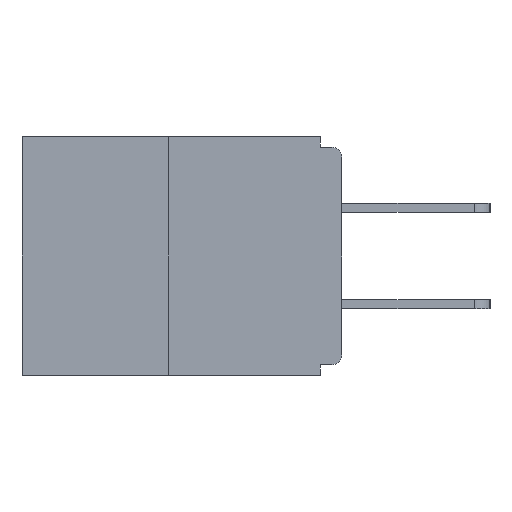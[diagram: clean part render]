
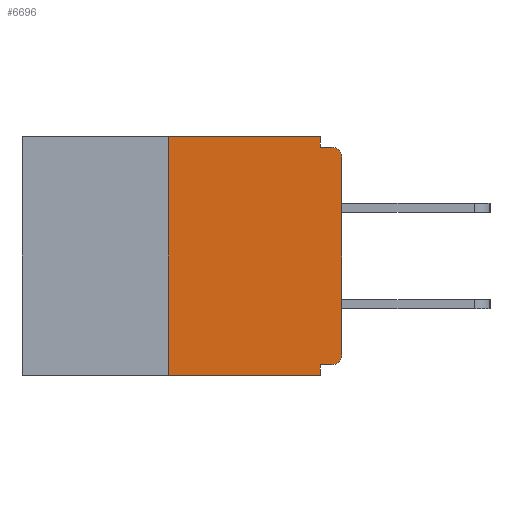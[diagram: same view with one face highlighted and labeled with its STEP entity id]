
A CAD part, left-side view. The second image highlights one B-rep face of the part: STEP entity #6696.
In plain terms, the highlighted planar face has unit normal (-1, 0, 0).
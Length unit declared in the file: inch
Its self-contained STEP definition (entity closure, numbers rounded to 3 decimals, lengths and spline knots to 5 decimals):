
#80 = FACE_OUTER_BOUND ( 'NONE', #8025, .T. ) ;
#126 = AXIS2_PLACEMENT_3D ( 'NONE', #13518, #20785, #20862 ) ;
#1583 = VECTOR ( 'NONE', #13262, 39.37008 ) ;
#1648 = EDGE_CURVE ( 'NONE', #8366, #12127, #14051, .T. ) ;
#1692 = CARTESIAN_POINT ( 'NONE',  ( 0., 0.031, -0.343 ) ) ;
#2750 = CIRCLE ( 'NONE', #5619, 0.015 ) ;
#3290 = LINE ( 'NONE', #3597, #17749 ) ;
#3597 = CARTESIAN_POINT ( 'NONE',  ( 0., 0.46, 0. ) ) ;
#3737 = CARTESIAN_POINT ( 'NONE',  ( 0., 0.25, 0. ) ) ;
#4111 = DIRECTION ( 'NONE',  ( 0., 0., 1. ) ) ;
#4221 = ORIENTED_EDGE ( 'NONE', *, *, #6422, .T. ) ;
#4353 = VECTOR ( 'NONE', #4111, 39.37008 ) ;
#4705 = VECTOR ( 'NONE', #17121, 39.37008 ) ;
#5236 = DIRECTION ( 'NONE',  ( 0., 1., 0. ) ) ;
#5619 = AXIS2_PLACEMENT_3D ( 'NONE', #15992, #16230, #19916 ) ;
#6003 = CARTESIAN_POINT ( 'NONE',  ( 0., 0., -0.03 ) ) ;
#6129 = CARTESIAN_POINT ( 'NONE',  ( 0., 0.031, 0. ) ) ;
#6188 = DIRECTION ( 'NONE',  ( 1., 0., 0. ) ) ;
#6380 = ORIENTED_EDGE ( 'NONE', *, *, #18710, .T. ) ;
#6422 = EDGE_CURVE ( 'NONE', #10304, #13069, #2750, .T. ) ;
#6431 = LINE ( 'NONE', #13459, #4353 ) ;
#6696 = ADVANCED_FACE ( 'NONE', ( #80 ), #14452, .F. ) ;
#7103 = CARTESIAN_POINT ( 'NONE',  ( 0., 0.46, 0. ) ) ;
#7266 = EDGE_CURVE ( 'NONE', #14106, #8366, #3290, .T. ) ;
#7717 = ORIENTED_EDGE ( 'NONE', *, *, #17049, .F. ) ;
#7814 = EDGE_CURVE ( 'NONE', #12127, #23131, #19762, .T. ) ;
#7955 = CARTESIAN_POINT ( 'NONE',  ( 0., 0.25, -0.343 ) ) ;
#8025 = EDGE_LOOP ( 'NONE', ( #20714, #7717, #24101, #23277, #8688, #4221, #6380, #9893, #10902, #16545 ) ) ;
#8089 = LINE ( 'NONE', #1692, #1583 ) ;
#8366 = VERTEX_POINT ( 'NONE', #6129 ) ;
#8688 = ORIENTED_EDGE ( 'NONE', *, *, #16845, .F. ) ;
#9039 = VECTOR ( 'NONE', #13764, 39.37008 ) ;
#9445 = LINE ( 'NONE', #14586, #22072 ) ;
#9713 = VERTEX_POINT ( 'NONE', #6003 ) ;
#9893 = ORIENTED_EDGE ( 'NONE', *, *, #14125, .T. ) ;
#10304 = VERTEX_POINT ( 'NONE', #21838 ) ;
#10309 = VERTEX_POINT ( 'NONE', #10747 ) ;
#10747 = CARTESIAN_POINT ( 'NONE',  ( 0., 0.031, -0.328 ) ) ;
#10902 = ORIENTED_EDGE ( 'NONE', *, *, #7814, .F. ) ;
#11762 = VERTEX_POINT ( 'NONE', #18087 ) ;
#12127 = VERTEX_POINT ( 'NONE', #23753 ) ;
#12614 = DIRECTION ( 'NONE',  ( 0., -1., 0. ) ) ;
#12662 = LINE ( 'NONE', #3737, #4705 ) ;
#12934 = AXIS2_PLACEMENT_3D ( 'NONE', #7103, #6188, #13776 ) ;
#13069 = VERTEX_POINT ( 'NONE', #16155 ) ;
#13191 = EDGE_CURVE ( 'NONE', #17833, #11762, #21735, .T. ) ;
#13262 = DIRECTION ( 'NONE',  ( 0., 0., -1. ) ) ;
#13459 = CARTESIAN_POINT ( 'NONE',  ( 0., 0., 0. ) ) ;
#13518 = CARTESIAN_POINT ( 'NONE',  ( 0., 0.015, -0.03 ) ) ;
#13764 = DIRECTION ( 'NONE',  ( 0., 0., -1. ) ) ;
#13776 = DIRECTION ( 'NONE',  ( 0., 0., -1. ) ) ;
#14051 = LINE ( 'NONE', #16008, #9039 ) ;
#14106 = VERTEX_POINT ( 'NONE', #22846 ) ;
#14125 = EDGE_CURVE ( 'NONE', #9713, #23131, #19913, .T. ) ;
#14452 = PLANE ( 'NONE',  #12934 ) ;
#14531 = EDGE_CURVE ( 'NONE', #10309, #11762, #8089, .T. ) ;
#14586 = CARTESIAN_POINT ( 'NONE',  ( 0., 0., -0.328 ) ) ;
#14615 = DIRECTION ( 'NONE',  ( 0., -1., 0. ) ) ;
#14805 = VECTOR ( 'NONE', #12614, 39.37008 ) ;
#15992 = CARTESIAN_POINT ( 'NONE',  ( 0., 0.015, -0.313 ) ) ;
#16008 = CARTESIAN_POINT ( 'NONE',  ( 0., 0.031, 0. ) ) ;
#16155 = CARTESIAN_POINT ( 'NONE',  ( 0., 0., -0.313 ) ) ;
#16230 = DIRECTION ( 'NONE',  ( -1., 0., 0. ) ) ;
#16545 = ORIENTED_EDGE ( 'NONE', *, *, #1648, .F. ) ;
#16845 = EDGE_CURVE ( 'NONE', #10304, #10309, #9445, .T. ) ;
#17049 = EDGE_CURVE ( 'NONE', #17833, #14106, #12662, .T. ) ;
#17121 = DIRECTION ( 'NONE',  ( 0., 0., 1. ) ) ;
#17749 = VECTOR ( 'NONE', #20743, 39.37008 ) ;
#17833 = VERTEX_POINT ( 'NONE', #7955 ) ;
#18087 = CARTESIAN_POINT ( 'NONE',  ( 0., 0.031, -0.343 ) ) ;
#18710 = EDGE_CURVE ( 'NONE', #13069, #9713, #6431, .T. ) ;
#19762 = LINE ( 'NONE', #21994, #14805 ) ;
#19913 = CIRCLE ( 'NONE', #126, 0.015 ) ;
#19916 = DIRECTION ( 'NONE',  ( 0., 0., -1. ) ) ;
#20177 = CARTESIAN_POINT ( 'NONE',  ( 0., 0.015, -0.015 ) ) ;
#20714 = ORIENTED_EDGE ( 'NONE', *, *, #7266, .F. ) ;
#20743 = DIRECTION ( 'NONE',  ( 0., -1., 0. ) ) ;
#20785 = DIRECTION ( 'NONE',  ( -1., 0., 0. ) ) ;
#20862 = DIRECTION ( 'NONE',  ( 0., 0., -1. ) ) ;
#20878 = VECTOR ( 'NONE', #14615, 39.37008 ) ;
#21735 = LINE ( 'NONE', #22735, #20878 ) ;
#21838 = CARTESIAN_POINT ( 'NONE',  ( 0., 0.015, -0.328 ) ) ;
#21994 = CARTESIAN_POINT ( 'NONE',  ( 0., 0., -0.015 ) ) ;
#22072 = VECTOR ( 'NONE', #5236, 39.37008 ) ;
#22735 = CARTESIAN_POINT ( 'NONE',  ( 0., 0.46, -0.343 ) ) ;
#22846 = CARTESIAN_POINT ( 'NONE',  ( 0., 0.25, 0. ) ) ;
#23131 = VERTEX_POINT ( 'NONE', #20177 ) ;
#23277 = ORIENTED_EDGE ( 'NONE', *, *, #14531, .F. ) ;
#23753 = CARTESIAN_POINT ( 'NONE',  ( 0., 0.031, -0.015 ) ) ;
#24101 = ORIENTED_EDGE ( 'NONE', *, *, #13191, .T. ) ;
